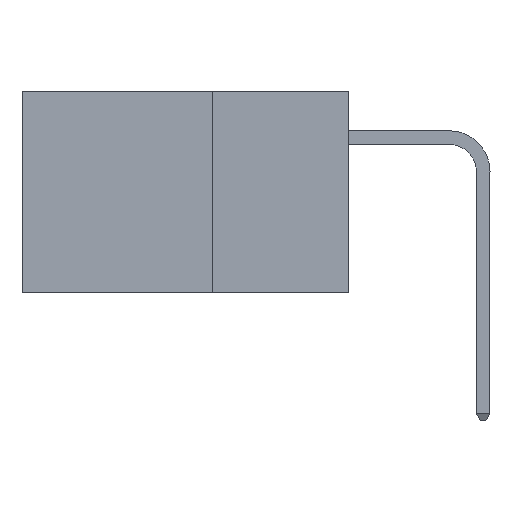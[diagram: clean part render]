
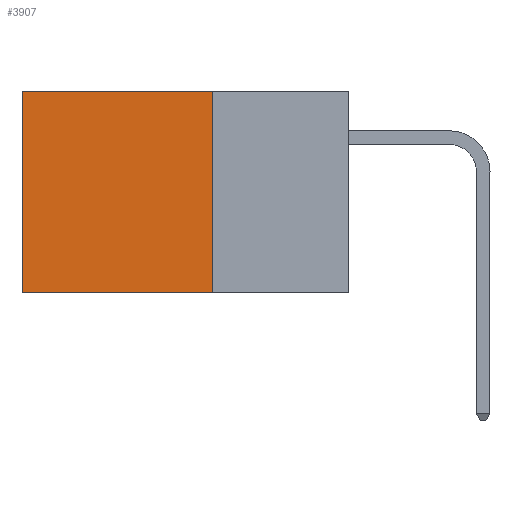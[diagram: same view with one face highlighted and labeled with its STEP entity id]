
A CAD part, left-side view. The second image highlights one B-rep face of the part: STEP entity #3907.
In plain terms, the highlighted planar face has unit normal (-1, 0, 0).
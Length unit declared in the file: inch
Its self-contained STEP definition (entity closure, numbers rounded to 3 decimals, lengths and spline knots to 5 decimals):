
#61 = DIRECTION ( 'NONE',  ( 0., 1., 0. ) ) ;
#540 = EDGE_LOOP ( 'NONE', ( #17779, #8382, #8949, #10995 ) ) ;
#1606 = CARTESIAN_POINT ( 'NONE',  ( 0.2875, 0.25, 0. ) ) ;
#1846 = CARTESIAN_POINT ( 'NONE',  ( 0.2875, 0.6, 0. ) ) ;
#2764 = LINE ( 'NONE', #25411, #18969 ) ;
#3465 = AXIS2_PLACEMENT_3D ( 'NONE', #16489, #20741, #8157 ) ;
#3807 = CARTESIAN_POINT ( 'NONE',  ( 0.2875, 0.6, -0.37 ) ) ;
#3907 = ADVANCED_FACE ( 'NONE', ( #10395 ), #26968, .F. ) ;
#4028 = DIRECTION ( 'NONE',  ( 0., 0., -1. ) ) ;
#4917 = DIRECTION ( 'NONE',  ( 0., 1., 0. ) ) ;
#6281 = LINE ( 'NONE', #19646, #16140 ) ;
#6863 = VECTOR ( 'NONE', #13717, 39.37008 ) ;
#8157 = DIRECTION ( 'NONE',  ( 0., 0., -1. ) ) ;
#8382 = ORIENTED_EDGE ( 'NONE', *, *, #22823, .F. ) ;
#8949 = ORIENTED_EDGE ( 'NONE', *, *, #24030, .F. ) ;
#9450 = EDGE_CURVE ( 'NONE', #10440, #10249, #2764, .T. ) ;
#10249 = VERTEX_POINT ( 'NONE', #19917 ) ;
#10395 = FACE_OUTER_BOUND ( 'NONE', #540, .T. ) ;
#10440 = VERTEX_POINT ( 'NONE', #1606 ) ;
#10995 = ORIENTED_EDGE ( 'NONE', *, *, #9450, .T. ) ;
#11636 = CARTESIAN_POINT ( 'NONE',  ( 0.2875, 0.25, 0. ) ) ;
#12444 = LINE ( 'NONE', #11636, #6863 ) ;
#12720 = VERTEX_POINT ( 'NONE', #18924 ) ;
#13341 = VECTOR ( 'NONE', #4028, 39.37008 ) ;
#13717 = DIRECTION ( 'NONE',  ( 0., 0., -1. ) ) ;
#16140 = VECTOR ( 'NONE', #4917, 39.37008 ) ;
#16489 = CARTESIAN_POINT ( 'NONE',  ( 0.2875, 0.25, 0. ) ) ;
#17779 = ORIENTED_EDGE ( 'NONE', *, *, #26102, .T. ) ;
#18924 = CARTESIAN_POINT ( 'NONE',  ( 0.2875, 0.25, -0.37 ) ) ;
#18946 = LINE ( 'NONE', #1846, #13341 ) ;
#18969 = VECTOR ( 'NONE', #61, 39.37008 ) ;
#19646 = CARTESIAN_POINT ( 'NONE',  ( 0.2875, 0.25, -0.37 ) ) ;
#19917 = CARTESIAN_POINT ( 'NONE',  ( 0.2875, 0.6, 0. ) ) ;
#20465 = VERTEX_POINT ( 'NONE', #3807 ) ;
#20741 = DIRECTION ( 'NONE',  ( 1., 0., 0. ) ) ;
#22823 = EDGE_CURVE ( 'NONE', #12720, #20465, #6281, .T. ) ;
#24030 = EDGE_CURVE ( 'NONE', #10440, #12720, #12444, .T. ) ;
#25411 = CARTESIAN_POINT ( 'NONE',  ( 0.2875, 0.25, 0. ) ) ;
#26102 = EDGE_CURVE ( 'NONE', #10249, #20465, #18946, .T. ) ;
#26968 = PLANE ( 'NONE',  #3465 ) ;
